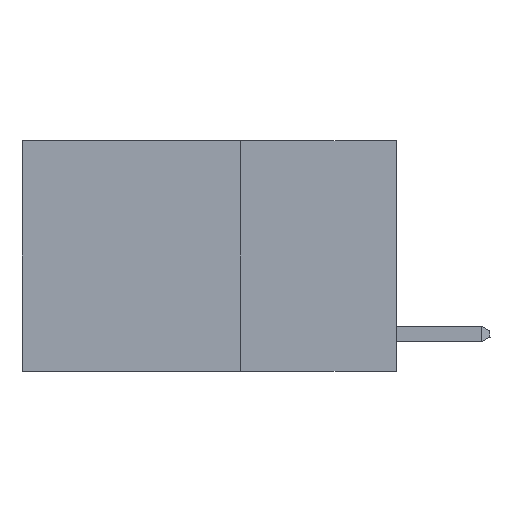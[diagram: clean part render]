
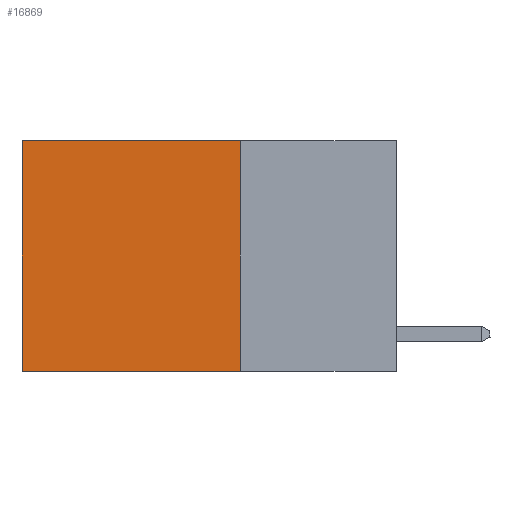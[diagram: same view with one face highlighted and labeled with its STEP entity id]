
A CAD part, left-side view. The second image highlights one B-rep face of the part: STEP entity #16869.
In plain terms, the highlighted planar face has unit normal (-1, 0, 0).
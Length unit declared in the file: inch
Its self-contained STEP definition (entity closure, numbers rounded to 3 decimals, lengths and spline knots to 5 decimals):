
#1244 = EDGE_CURVE ( 'NONE', #2278, #16877, #26996, .T. ) ;
#2278 = VERTEX_POINT ( 'NONE', #25339 ) ;
#2396 = DIRECTION ( 'NONE',  ( 0., 0., -1. ) ) ;
#4252 = EDGE_CURVE ( 'NONE', #16877, #13005, #10193, .T. ) ;
#4264 = DIRECTION ( 'NONE',  ( 0., 1., 0. ) ) ;
#4285 = EDGE_CURVE ( 'NONE', #2278, #9272, #14681, .T. ) ;
#5298 = LINE ( 'NONE', #19280, #24647 ) ;
#5623 = ORIENTED_EDGE ( 'NONE', *, *, #4285, .T. ) ;
#7368 = DIRECTION ( 'NONE',  ( 0., 0., -1. ) ) ;
#7410 = ORIENTED_EDGE ( 'NONE', *, *, #17395, .T. ) ;
#7748 = ORIENTED_EDGE ( 'NONE', *, *, #1244, .F. ) ;
#8113 = DIRECTION ( 'NONE',  ( 0., 1., 0. ) ) ;
#8122 = DIRECTION ( 'NONE',  ( 0., 0., -1. ) ) ;
#9272 = VERTEX_POINT ( 'NONE', #23862 ) ;
#10193 = LINE ( 'NONE', #12777, #26501 ) ;
#11308 = ORIENTED_EDGE ( 'NONE', *, *, #4252, .F. ) ;
#12243 = CARTESIAN_POINT ( 'NONE',  ( 0.2625, 0.25, 0. ) ) ;
#12777 = CARTESIAN_POINT ( 'NONE',  ( 0.2625, 0.25, -0.37 ) ) ;
#13005 = VERTEX_POINT ( 'NONE', #15865 ) ;
#13419 = VECTOR ( 'NONE', #4264, 39.37008 ) ;
#14681 = LINE ( 'NONE', #23007, #13419 ) ;
#15865 = CARTESIAN_POINT ( 'NONE',  ( 0.2625, 0.6, -0.37 ) ) ;
#16869 = ADVANCED_FACE ( 'NONE', ( #22622 ), #25069, .F. ) ;
#16877 = VERTEX_POINT ( 'NONE', #20992 ) ;
#17222 = AXIS2_PLACEMENT_3D ( 'NONE', #12243, #18538, #8122 ) ;
#17395 = EDGE_CURVE ( 'NONE', #9272, #13005, #5298, .T. ) ;
#18538 = DIRECTION ( 'NONE',  ( 1., 0., 0. ) ) ;
#19280 = CARTESIAN_POINT ( 'NONE',  ( 0.2625, 0.6, 0. ) ) ;
#20992 = CARTESIAN_POINT ( 'NONE',  ( 0.2625, 0.25, -0.37 ) ) ;
#22222 = EDGE_LOOP ( 'NONE', ( #7410, #11308, #7748, #5623 ) ) ;
#22622 = FACE_OUTER_BOUND ( 'NONE', #22222, .T. ) ;
#23007 = CARTESIAN_POINT ( 'NONE',  ( 0.2625, 0.25, 0. ) ) ;
#23862 = CARTESIAN_POINT ( 'NONE',  ( 0.2625, 0.6, 0. ) ) ;
#23894 = VECTOR ( 'NONE', #2396, 39.37008 ) ;
#24647 = VECTOR ( 'NONE', #7368, 39.37008 ) ;
#25069 = PLANE ( 'NONE',  #17222 ) ;
#25339 = CARTESIAN_POINT ( 'NONE',  ( 0.2625, 0.25, 0. ) ) ;
#25370 = CARTESIAN_POINT ( 'NONE',  ( 0.2625, 0.25, 0. ) ) ;
#26501 = VECTOR ( 'NONE', #8113, 39.37008 ) ;
#26996 = LINE ( 'NONE', #25370, #23894 ) ;
